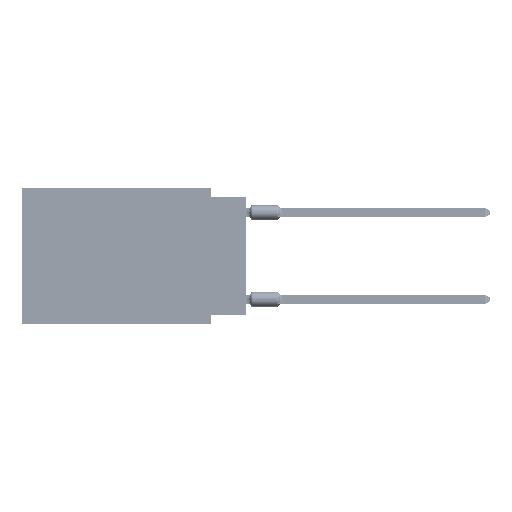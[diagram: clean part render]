
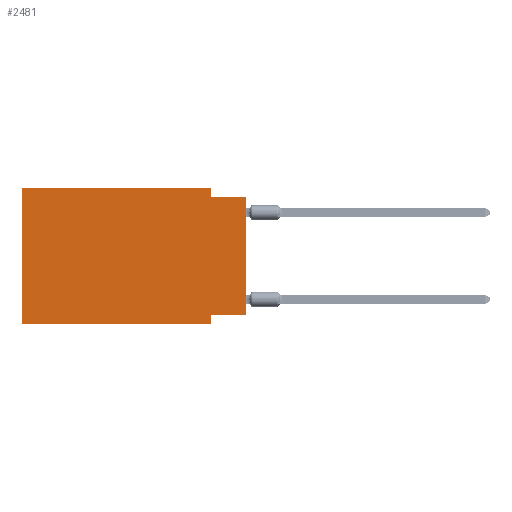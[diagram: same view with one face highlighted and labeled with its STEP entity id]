
A CAD part, left-side view. The second image highlights one B-rep face of the part: STEP entity #2481.
In plain terms, the highlighted planar face has unit normal (-1, 0, 0).
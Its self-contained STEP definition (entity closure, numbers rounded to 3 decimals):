
#449 = CARTESIAN_POINT ( 'NONE',  ( 0., 2.54, 0. ) ) ;
#2481 = ADVANCED_FACE ( 'NONE', ( #54639 ), #34019, .F. ) ;
#8236 = CARTESIAN_POINT ( 'NONE',  ( 0., 16.383, 0. ) ) ;
#9305 = ORIENTED_EDGE ( 'NONE', *, *, #45983, .F. ) ;
#10257 = VECTOR ( 'NONE', #48645, 1000. ) ;
#11061 = ORIENTED_EDGE ( 'NONE', *, *, #77605, .F. ) ;
#11906 = CARTESIAN_POINT ( 'NONE',  ( 0., 0., 0. ) ) ;
#13028 = CARTESIAN_POINT ( 'NONE',  ( 0., 0., -9.271 ) ) ;
#13407 = LINE ( 'NONE', #13028, #68871 ) ;
#13821 = EDGE_CURVE ( 'NONE', #33533, #42098, #41860, .T. ) ;
#13868 = EDGE_CURVE ( 'NONE', #36476, #28645, #66573, .T. ) ;
#14305 = EDGE_CURVE ( 'NONE', #36476, #44948, #13407, .T. ) ;
#14611 = AXIS2_PLACEMENT_3D ( 'NONE', #34008, #21627, #28010 ) ;
#15329 = VERTEX_POINT ( 'NONE', #59039 ) ;
#18967 = DIRECTION ( 'NONE',  ( 0., 0., 1. ) ) ;
#19527 = VERTEX_POINT ( 'NONE', #449 ) ;
#20707 = ORIENTED_EDGE ( 'NONE', *, *, #35498, .F. ) ;
#21627 = DIRECTION ( 'NONE',  ( 1., 0., 0. ) ) ;
#23892 = DIRECTION ( 'NONE',  ( 0., -1., 0. ) ) ;
#28010 = DIRECTION ( 'NONE',  ( 0., 0., -1. ) ) ;
#28051 = LINE ( 'NONE', #51633, #77990 ) ;
#28645 = VERTEX_POINT ( 'NONE', #54315 ) ;
#29077 = DIRECTION ( 'NONE',  ( 0., 0., -1. ) ) ;
#29305 = CARTESIAN_POINT ( 'NONE',  ( 0., 2.54, -9.271 ) ) ;
#30725 = LINE ( 'NONE', #43086, #42113 ) ;
#33533 = VERTEX_POINT ( 'NONE', #56589 ) ;
#34008 = CARTESIAN_POINT ( 'NONE',  ( 0., 16.383, 0. ) ) ;
#34019 = PLANE ( 'NONE',  #14611 ) ;
#34688 = LINE ( 'NONE', #60212, #44094 ) ;
#34835 = DIRECTION ( 'NONE',  ( 0., -1., 0. ) ) ;
#35498 = EDGE_CURVE ( 'NONE', #70481, #19527, #78743, .T. ) ;
#36476 = VERTEX_POINT ( 'NONE', #75439 ) ;
#36987 = DIRECTION ( 'NONE',  ( 0., 1., 0. ) ) ;
#40564 = EDGE_CURVE ( 'NONE', #33533, #70481, #61310, .T. ) ;
#41268 = CARTESIAN_POINT ( 'NONE',  ( 0., 2.54, -9.906 ) ) ;
#41860 = LINE ( 'NONE', #66179, #67517 ) ;
#42098 = VERTEX_POINT ( 'NONE', #41268 ) ;
#42113 = VECTOR ( 'NONE', #67408, 1000. ) ;
#43086 = CARTESIAN_POINT ( 'NONE',  ( 0., 2.54, -9.906 ) ) ;
#43355 = CARTESIAN_POINT ( 'NONE',  ( 0., 16.383, 0. ) ) ;
#44094 = VECTOR ( 'NONE', #29077, 1000. ) ;
#44948 = VERTEX_POINT ( 'NONE', #29305 ) ;
#45983 = EDGE_CURVE ( 'NONE', #44948, #42098, #30725, .T. ) ;
#46131 = VECTOR ( 'NONE', #72358, 1000. ) ;
#47775 = ORIENTED_EDGE ( 'NONE', *, *, #13821, .T. ) ;
#48645 = DIRECTION ( 'NONE',  ( 0., 0., 1. ) ) ;
#50135 = EDGE_CURVE ( 'NONE', #15329, #28645, #28051, .T. ) ;
#50995 = ORIENTED_EDGE ( 'NONE', *, *, #14305, .F. ) ;
#51593 = ORIENTED_EDGE ( 'NONE', *, *, #13868, .T. ) ;
#51633 = CARTESIAN_POINT ( 'NONE',  ( 0., 0., -0.635 ) ) ;
#52191 = ORIENTED_EDGE ( 'NONE', *, *, #40564, .F. ) ;
#54315 = CARTESIAN_POINT ( 'NONE',  ( 0., 0., -0.635 ) ) ;
#54639 = FACE_OUTER_BOUND ( 'NONE', #67021, .T. ) ;
#56589 = CARTESIAN_POINT ( 'NONE',  ( 0., 16.383, -9.906 ) ) ;
#59039 = CARTESIAN_POINT ( 'NONE',  ( 0., 2.54, -0.635 ) ) ;
#59393 = VECTOR ( 'NONE', #18967, 1000. ) ;
#60212 = CARTESIAN_POINT ( 'NONE',  ( 0., 2.54, 0. ) ) ;
#60444 = CARTESIAN_POINT ( 'NONE',  ( 0., 16.383, 0. ) ) ;
#61310 = LINE ( 'NONE', #43355, #59393 ) ;
#66179 = CARTESIAN_POINT ( 'NONE',  ( 0., 16.383, -9.906 ) ) ;
#66573 = LINE ( 'NONE', #11906, #10257 ) ;
#67021 = EDGE_LOOP ( 'NONE', ( #51593, #77584, #11061, #20707, #52191, #47775, #9305, #50995 ) ) ;
#67408 = DIRECTION ( 'NONE',  ( 0., 0., -1. ) ) ;
#67517 = VECTOR ( 'NONE', #23892, 1000. ) ;
#68871 = VECTOR ( 'NONE', #36987, 1000. ) ;
#70481 = VERTEX_POINT ( 'NONE', #8236 ) ;
#72358 = DIRECTION ( 'NONE',  ( 0., -1., 0. ) ) ;
#75439 = CARTESIAN_POINT ( 'NONE',  ( 0., 0., -9.271 ) ) ;
#77584 = ORIENTED_EDGE ( 'NONE', *, *, #50135, .F. ) ;
#77605 = EDGE_CURVE ( 'NONE', #19527, #15329, #34688, .T. ) ;
#77990 = VECTOR ( 'NONE', #34835, 1000. ) ;
#78743 = LINE ( 'NONE', #60444, #46131 ) ;
